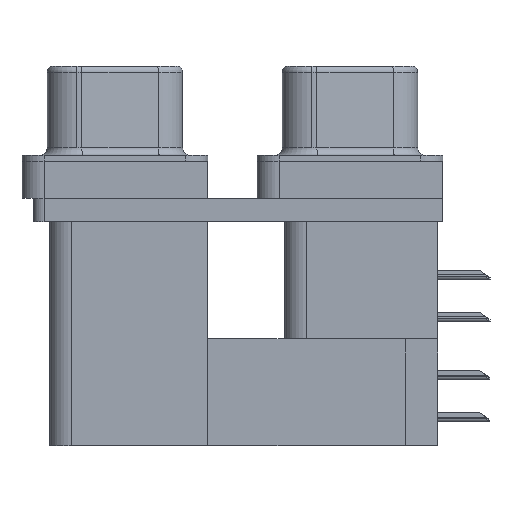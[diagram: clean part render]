
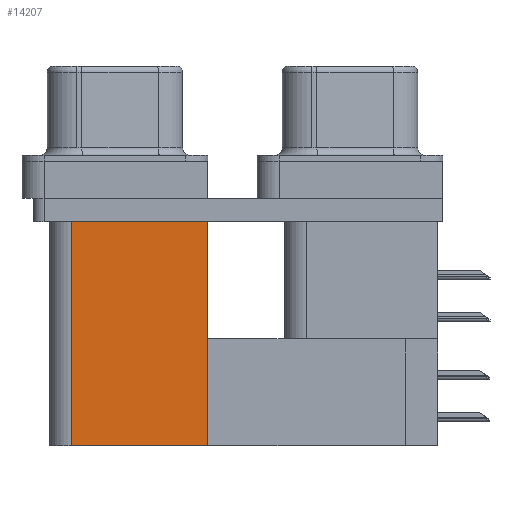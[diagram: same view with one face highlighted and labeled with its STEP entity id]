
A CAD part, left-side view. The second image highlights one B-rep face of the part: STEP entity #14207.
In plain terms, the highlighted planar face has unit normal (-1, 0, 0).
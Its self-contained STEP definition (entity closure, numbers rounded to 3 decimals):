
#344 = DIRECTION ( 'NONE',  ( 0., 1., 0. ) ) ;
#466 = DIRECTION ( 'NONE',  ( 0., 0., -1. ) ) ;
#1033 = FACE_OUTER_BOUND ( 'NONE', #11976, .T. ) ;
#1248 = VERTEX_POINT ( 'NONE', #21587 ) ;
#2394 = CARTESIAN_POINT ( 'NONE',  ( 3.7, 18.8, -19.2 ) ) ;
#3220 = VERTEX_POINT ( 'NONE', #36988 ) ;
#3620 = AXIS2_PLACEMENT_3D ( 'NONE', #23804, #26478, #466 ) ;
#5660 = CARTESIAN_POINT ( 'NONE',  ( 3.7, 9.6, -2.5 ) ) ;
#11900 = LINE ( 'NONE', #5660, #26707 ) ;
#11976 = EDGE_LOOP ( 'NONE', ( #36544, #34117, #26907, #31064 ) ) ;
#13285 = CARTESIAN_POINT ( 'NONE',  ( 3.7, 9.6, -19.2 ) ) ;
#14207 = ADVANCED_FACE ( 'NONE', ( #1033 ), #23617, .F. ) ;
#17322 = EDGE_CURVE ( 'NONE', #1248, #3220, #33421, .T. ) ;
#17468 = EDGE_CURVE ( 'NONE', #1248, #25760, #22779, .T. ) ;
#17577 = DIRECTION ( 'NONE',  ( 0., 0., 1. ) ) ;
#17765 = VECTOR ( 'NONE', #18991, 1000. ) ;
#18991 = DIRECTION ( 'NONE',  ( 0., 0., 1. ) ) ;
#21131 = EDGE_CURVE ( 'NONE', #3220, #30072, #11900, .T. ) ;
#21587 = CARTESIAN_POINT ( 'NONE',  ( 3.7, 9.6, -19.2 ) ) ;
#22213 = CARTESIAN_POINT ( 'NONE',  ( 3.7, 18.8, -2.5 ) ) ;
#22779 = LINE ( 'NONE', #31128, #31719 ) ;
#23617 = PLANE ( 'NONE',  #3620 ) ;
#23804 = CARTESIAN_POINT ( 'NONE',  ( 3.7, 9.6, -19.2 ) ) ;
#25760 = VERTEX_POINT ( 'NONE', #2394 ) ;
#26478 = DIRECTION ( 'NONE',  ( 1., 0., 0. ) ) ;
#26707 = VECTOR ( 'NONE', #344, 1000. ) ;
#26907 = ORIENTED_EDGE ( 'NONE', *, *, #17468, .F. ) ;
#29148 = LINE ( 'NONE', #29331, #31148 ) ;
#29331 = CARTESIAN_POINT ( 'NONE',  ( 3.7, 18.8, -19.2 ) ) ;
#29433 = EDGE_CURVE ( 'NONE', #25760, #30072, #29148, .T. ) ;
#30072 = VERTEX_POINT ( 'NONE', #22213 ) ;
#31064 = ORIENTED_EDGE ( 'NONE', *, *, #17322, .T. ) ;
#31128 = CARTESIAN_POINT ( 'NONE',  ( 3.7, 9.6, -19.2 ) ) ;
#31148 = VECTOR ( 'NONE', #17577, 1000. ) ;
#31509 = DIRECTION ( 'NONE',  ( 0., 1., 0. ) ) ;
#31719 = VECTOR ( 'NONE', #31509, 1000. ) ;
#33421 = LINE ( 'NONE', #13285, #17765 ) ;
#34117 = ORIENTED_EDGE ( 'NONE', *, *, #29433, .F. ) ;
#36544 = ORIENTED_EDGE ( 'NONE', *, *, #21131, .T. ) ;
#36988 = CARTESIAN_POINT ( 'NONE',  ( 3.7, 9.6, -2.5 ) ) ;
